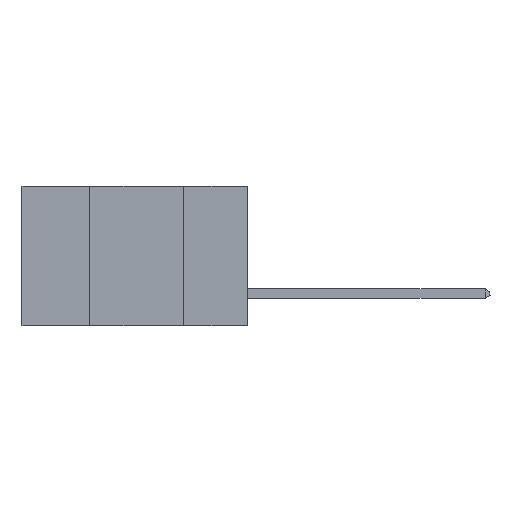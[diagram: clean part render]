
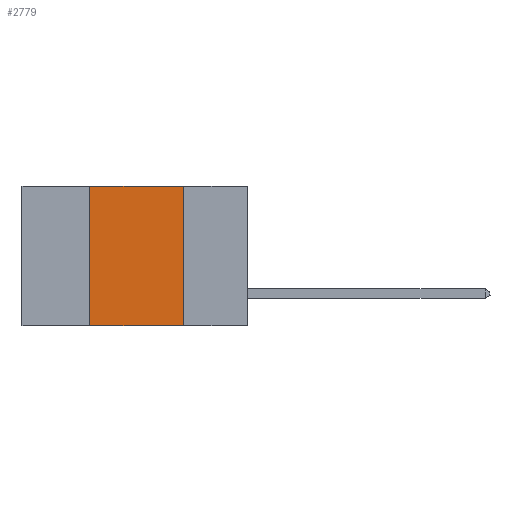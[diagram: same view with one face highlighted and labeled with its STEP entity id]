
A CAD part, left-side view. The second image highlights one B-rep face of the part: STEP entity #2779.
In plain terms, the highlighted planar face has unit normal (-1, 0, 0).
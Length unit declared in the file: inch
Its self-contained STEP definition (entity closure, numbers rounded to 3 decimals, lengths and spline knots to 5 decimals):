
#2779 = ADVANCED_FACE ( 'NONE', ( #14603 ), #23727, .F. ) ;
#3334 = DIRECTION ( 'NONE',  ( 0., -1., 0. ) ) ;
#3647 = VERTEX_POINT ( 'NONE', #5206 ) ;
#5206 = CARTESIAN_POINT ( 'NONE',  ( 0., 0.42, -0.37 ) ) ;
#5528 = ORIENTED_EDGE ( 'NONE', *, *, #20221, .T. ) ;
#5637 = VERTEX_POINT ( 'NONE', #10348 ) ;
#5971 = CARTESIAN_POINT ( 'NONE',  ( 0., 0.6, 0. ) ) ;
#6033 = EDGE_CURVE ( 'NONE', #3647, #8686, #9145, .T. ) ;
#6255 = VECTOR ( 'NONE', #12072, 39.37008 ) ;
#6308 = VERTEX_POINT ( 'NONE', #14566 ) ;
#7071 = CARTESIAN_POINT ( 'NONE',  ( 0., 0.42, 0. ) ) ;
#8686 = VERTEX_POINT ( 'NONE', #7071 ) ;
#9145 = LINE ( 'NONE', #22557, #23089 ) ;
#9948 = CARTESIAN_POINT ( 'NONE',  ( 0., 0.6, -0.37 ) ) ;
#10239 = DIRECTION ( 'NONE',  ( 1., 0., 0. ) ) ;
#10332 = DIRECTION ( 'NONE',  ( 0., 0., -1. ) ) ;
#10348 = CARTESIAN_POINT ( 'NONE',  ( 0., 0.17, -0.37 ) ) ;
#11303 = DIRECTION ( 'NONE',  ( 0., 0., -1. ) ) ;
#11522 = ORIENTED_EDGE ( 'NONE', *, *, #21686, .F. ) ;
#12072 = DIRECTION ( 'NONE',  ( 0., -1., 0. ) ) ;
#14566 = CARTESIAN_POINT ( 'NONE',  ( 0., 0.17, 0. ) ) ;
#14603 = FACE_OUTER_BOUND ( 'NONE', #16342, .T. ) ;
#15221 = VECTOR ( 'NONE', #11303, 39.37008 ) ;
#16342 = EDGE_LOOP ( 'NONE', ( #11522, #28935, #17151, #5528 ) ) ;
#16552 = DIRECTION ( 'NONE',  ( 0., 0., 1. ) ) ;
#17151 = ORIENTED_EDGE ( 'NONE', *, *, #6033, .F. ) ;
#19982 = LINE ( 'NONE', #5971, #20307 ) ;
#20221 = EDGE_CURVE ( 'NONE', #3647, #5637, #25381, .T. ) ;
#20307 = VECTOR ( 'NONE', #3334, 39.37008 ) ;
#21096 = LINE ( 'NONE', #22175, #15221 ) ;
#21686 = EDGE_CURVE ( 'NONE', #6308, #5637, #21096, .T. ) ;
#22175 = CARTESIAN_POINT ( 'NONE',  ( 0., 0.17, 0. ) ) ;
#22557 = CARTESIAN_POINT ( 'NONE',  ( 0., 0.42, 0. ) ) ;
#22558 = EDGE_CURVE ( 'NONE', #8686, #6308, #19982, .T. ) ;
#23089 = VECTOR ( 'NONE', #16552, 39.37008 ) ;
#23727 = PLANE ( 'NONE',  #27141 ) ;
#25381 = LINE ( 'NONE', #9948, #6255 ) ;
#25864 = CARTESIAN_POINT ( 'NONE',  ( 0., 0.6, 0. ) ) ;
#27141 = AXIS2_PLACEMENT_3D ( 'NONE', #25864, #10239, #10332 ) ;
#28935 = ORIENTED_EDGE ( 'NONE', *, *, #22558, .F. ) ;
